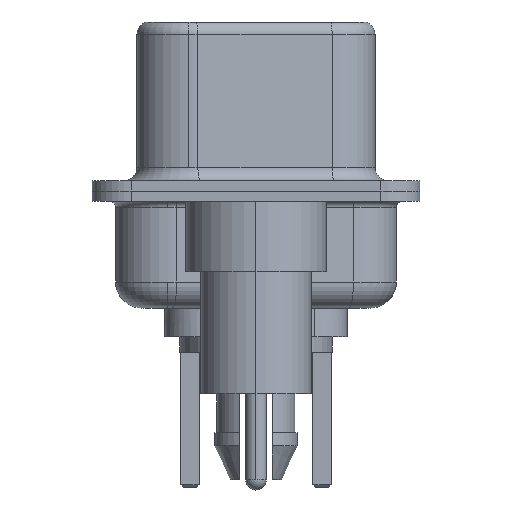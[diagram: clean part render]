
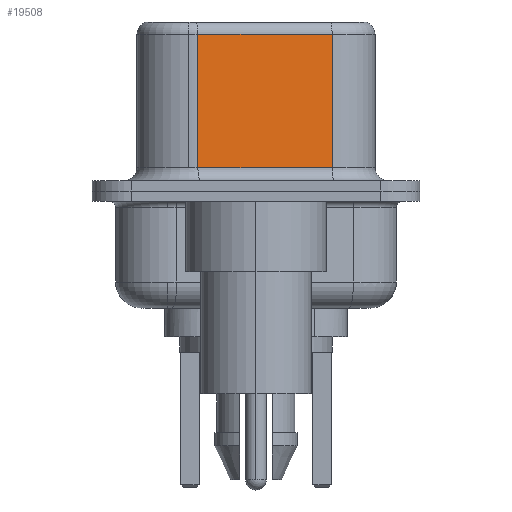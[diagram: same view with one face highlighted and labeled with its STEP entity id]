
A CAD part, left-side view. The second image highlights one B-rep face of the part: STEP entity #19508.
In plain terms, the highlighted planar face has unit normal (-0.985, -0.174, 0).
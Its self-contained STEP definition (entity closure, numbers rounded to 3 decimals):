
#305 = VECTOR ( 'NONE', #14023, 1000. ) ;
#1432 = LINE ( 'NONE', #22897, #305 ) ;
#1575 = VECTOR ( 'NONE', #11304, 1000. ) ;
#2810 = DIRECTION ( 'NONE',  ( 0., 0., -1. ) ) ;
#2908 = VERTEX_POINT ( 'NONE', #6509 ) ;
#3154 = LINE ( 'NONE', #13633, #11558 ) ;
#4511 = PLANE ( 'NONE',  #16172 ) ;
#4512 = ORIENTED_EDGE ( 'NONE', *, *, #17206, .F. ) ;
#6405 = DIRECTION ( 'NONE',  ( 0.985, 0.174, 0. ) ) ;
#6509 = CARTESIAN_POINT ( 'NONE',  ( 4.58, -2.927, 0.9 ) ) ;
#6765 = VECTOR ( 'NONE', #13157, 1000. ) ;
#7632 = CARTESIAN_POINT ( 'NONE',  ( 4.58, -2.927, 6.02 ) ) ;
#7912 = VERTEX_POINT ( 'NONE', #14047 ) ;
#8141 = CARTESIAN_POINT ( 'NONE',  ( 4.58, -2.927, 6.52 ) ) ;
#8464 = CARTESIAN_POINT ( 'NONE',  ( 4.58, -2.927, 6.02 ) ) ;
#9490 = CARTESIAN_POINT ( 'NONE',  ( 4.58, -2.927, 6.52 ) ) ;
#9815 = EDGE_CURVE ( 'NONE', #13063, #7912, #3154, .T. ) ;
#9960 = EDGE_CURVE ( 'NONE', #7912, #2908, #1432, .T. ) ;
#10536 = ORIENTED_EDGE ( 'NONE', *, *, #9960, .T. ) ;
#11304 = DIRECTION ( 'NONE',  ( -0.174, 0.985, 0. ) ) ;
#11539 = LINE ( 'NONE', #9490, #6765 ) ;
#11558 = VECTOR ( 'NONE', #2810, 1000. ) ;
#11664 = VERTEX_POINT ( 'NONE', #8464 ) ;
#11965 = CARTESIAN_POINT ( 'NONE',  ( 3.67, 2.233, 6.02 ) ) ;
#12569 = EDGE_LOOP ( 'NONE', ( #4512, #12882, #17839, #10536 ) ) ;
#12882 = ORIENTED_EDGE ( 'NONE', *, *, #20682, .T. ) ;
#13063 = VERTEX_POINT ( 'NONE', #11965 ) ;
#13157 = DIRECTION ( 'NONE',  ( 0., 0., -1. ) ) ;
#13633 = CARTESIAN_POINT ( 'NONE',  ( 3.67, 2.233, 6.52 ) ) ;
#14023 = DIRECTION ( 'NONE',  ( 0.174, -0.985, 0. ) ) ;
#14047 = CARTESIAN_POINT ( 'NONE',  ( 3.67, 2.233, 0.9 ) ) ;
#14918 = FACE_OUTER_BOUND ( 'NONE', #12569, .T. ) ;
#16172 = AXIS2_PLACEMENT_3D ( 'NONE', #8141, #6405, #18987 ) ;
#17206 = EDGE_CURVE ( 'NONE', #11664, #2908, #11539, .T. ) ;
#17839 = ORIENTED_EDGE ( 'NONE', *, *, #9815, .T. ) ;
#18987 = DIRECTION ( 'NONE',  ( -0.174, 0.985, 0. ) ) ;
#19508 = ADVANCED_FACE ( 'NONE', ( #14918 ), #4511, .F. ) ;
#20682 = EDGE_CURVE ( 'NONE', #11664, #13063, #20686, .T. ) ;
#20686 = LINE ( 'NONE', #7632, #1575 ) ;
#22897 = CARTESIAN_POINT ( 'NONE',  ( 4.58, -2.927, 0.9 ) ) ;
